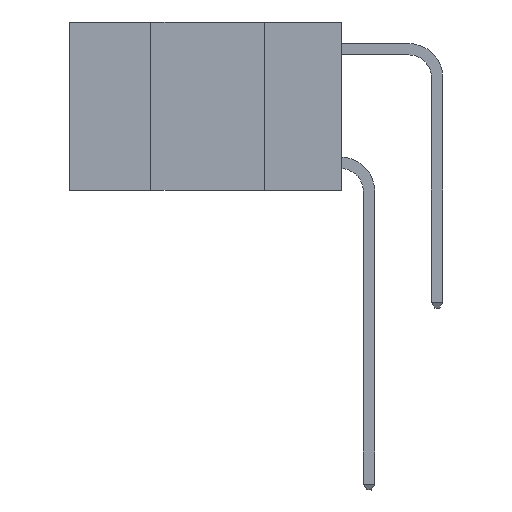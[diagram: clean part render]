
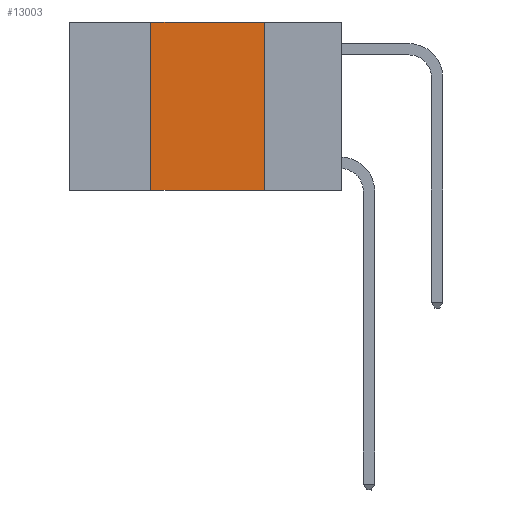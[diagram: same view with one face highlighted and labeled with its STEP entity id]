
A CAD part, left-side view. The second image highlights one B-rep face of the part: STEP entity #13003.
In plain terms, the highlighted planar face has unit normal (-1, 0, 0).
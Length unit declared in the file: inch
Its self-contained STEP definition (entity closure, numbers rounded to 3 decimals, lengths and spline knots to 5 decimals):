
#576 = EDGE_LOOP ( 'NONE', ( #9887, #10347, #3198, #18383 ) ) ;
#671 = CARTESIAN_POINT ( 'NONE',  ( 0., 0.42, 0. ) ) ;
#1224 = VECTOR ( 'NONE', #10936, 39.37008 ) ;
#2393 = EDGE_CURVE ( 'NONE', #8210, #8736, #6751, .T. ) ;
#3198 = ORIENTED_EDGE ( 'NONE', *, *, #5403, .F. ) ;
#4835 = CARTESIAN_POINT ( 'NONE',  ( 0., 0.6, -0.37 ) ) ;
#5282 = FACE_OUTER_BOUND ( 'NONE', #576, .T. ) ;
#5317 = VECTOR ( 'NONE', #6642, 39.37008 ) ;
#5403 = EDGE_CURVE ( 'NONE', #8210, #13707, #16493, .T. ) ;
#5757 = LINE ( 'NONE', #11016, #5317 ) ;
#6450 = PLANE ( 'NONE',  #18318 ) ;
#6642 = DIRECTION ( 'NONE',  ( 0., -1., 0. ) ) ;
#6751 = LINE ( 'NONE', #4835, #10150 ) ;
#7479 = CARTESIAN_POINT ( 'NONE',  ( 0., 0.42, -0.37 ) ) ;
#7943 = CARTESIAN_POINT ( 'NONE',  ( 0., 0.17, 0. ) ) ;
#8210 = VERTEX_POINT ( 'NONE', #7479 ) ;
#8736 = VERTEX_POINT ( 'NONE', #17285 ) ;
#9222 = LINE ( 'NONE', #7943, #13464 ) ;
#9357 = DIRECTION ( 'NONE',  ( 0., 0., -1. ) ) ;
#9500 = CARTESIAN_POINT ( 'NONE',  ( 0., 0.42, 0. ) ) ;
#9887 = ORIENTED_EDGE ( 'NONE', *, *, #18067, .F. ) ;
#9983 = CARTESIAN_POINT ( 'NONE',  ( 0., 0.17, 0. ) ) ;
#10150 = VECTOR ( 'NONE', #11978, 39.37008 ) ;
#10347 = ORIENTED_EDGE ( 'NONE', *, *, #12085, .F. ) ;
#10936 = DIRECTION ( 'NONE',  ( 0., 0., 1. ) ) ;
#11016 = CARTESIAN_POINT ( 'NONE',  ( 0., 0.6, 0. ) ) ;
#11978 = DIRECTION ( 'NONE',  ( 0., -1., 0. ) ) ;
#12085 = EDGE_CURVE ( 'NONE', #13707, #12784, #5757, .T. ) ;
#12784 = VERTEX_POINT ( 'NONE', #9983 ) ;
#13003 = ADVANCED_FACE ( 'NONE', ( #5282 ), #6450, .F. ) ;
#13464 = VECTOR ( 'NONE', #17947, 39.37008 ) ;
#13707 = VERTEX_POINT ( 'NONE', #671 ) ;
#16460 = CARTESIAN_POINT ( 'NONE',  ( 0., 0.6, 0. ) ) ;
#16493 = LINE ( 'NONE', #9500, #1224 ) ;
#17285 = CARTESIAN_POINT ( 'NONE',  ( 0., 0.17, -0.37 ) ) ;
#17918 = DIRECTION ( 'NONE',  ( 1., 0., 0. ) ) ;
#17947 = DIRECTION ( 'NONE',  ( 0., 0., -1. ) ) ;
#18067 = EDGE_CURVE ( 'NONE', #12784, #8736, #9222, .T. ) ;
#18318 = AXIS2_PLACEMENT_3D ( 'NONE', #16460, #17918, #9357 ) ;
#18383 = ORIENTED_EDGE ( 'NONE', *, *, #2393, .T. ) ;
